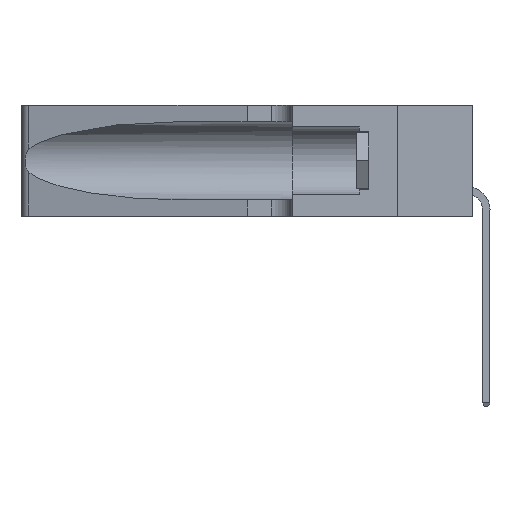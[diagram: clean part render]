
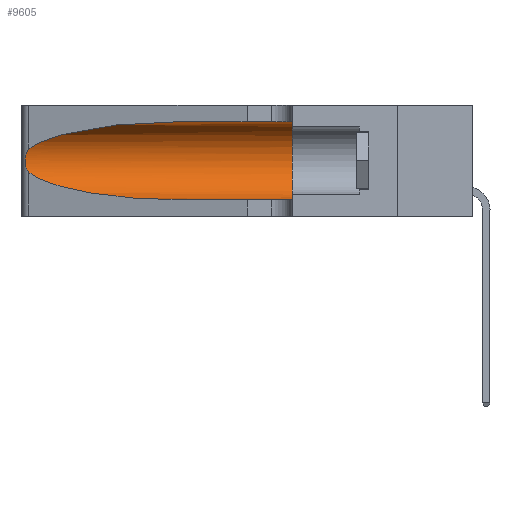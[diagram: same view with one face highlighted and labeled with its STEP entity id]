
A CAD part, left-side view. The second image highlights one B-rep face of the part: STEP entity #9605.
In plain terms, the highlighted cylindrical face has radius 3.308 mm (diameter 6.617 mm), a partial arc.
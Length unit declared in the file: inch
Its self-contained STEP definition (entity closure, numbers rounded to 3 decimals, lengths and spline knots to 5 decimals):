
#351 = CARTESIAN_POINT ( 'NONE',  ( 0.1305, 1.61858, 0.31525 ) ) ;
#369 = CARTESIAN_POINT ( 'NONE',  ( 0.18966, 0.96281, 0.05475 ) ) ;
#580 = VECTOR ( 'NONE', #4025, 39.37008 ) ;
#853 = CARTESIAN_POINT ( 'NONE',  ( 0.1305, 1.61858, 0.05475 ) ) ;
#1292 = CARTESIAN_POINT ( 'NONE',  ( 0.25555, 1.22994, 0.2215 ) ) ;
#1691 = CARTESIAN_POINT ( 'NONE',  ( 0.25487, 1.22718, 0.22369 ) ) ;
#1742 = B_SPLINE_CURVE_WITH_KNOTS ( 'NONE', 3,
 ( #2287, #1292, #12880, #4626, #5923, #19458, #17597, #19232, #20907, #10933, #14302, #15964, #11426, #6297 ),
 .UNSPECIFIED., .F., .F.,
 ( 4, 2, 2, 2, 2, 2, 4 ),
 ( 0., 0.00027, 0.00053, 0.00107, 0.0016, 0.00187, 0.00214 ),
 .UNSPECIFIED. ) ;
#1849 = DIRECTION ( 'NONE',  ( 0., 0., -1. ) ) ;
#1911 = DIRECTION ( 'NONE',  ( 0., -1., 0. ) ) ;
#1985 = CARTESIAN_POINT ( 'NONE',  ( 0.1305, 0.35, 0.05475 ) ) ;
#2013 = ORIENTED_EDGE ( 'NONE', *, *, #16988, .T. ) ;
#2097 = EDGE_CURVE ( 'NONE', #17819, #12978, #13311, .T. ) ;
#2272 = VERTEX_POINT ( 'NONE', #18849 ) ;
#2287 = CARTESIAN_POINT ( 'NONE',  ( 0.25487, 1.22718, 0.22369 ) ) ;
#2636 = ORIENTED_EDGE ( 'NONE', *, *, #2097, .F. ) ;
#3358 = CARTESIAN_POINT ( 'NONE',  ( 0.1305, 0.72297, 0.05475 ) ) ;
#3577 = EDGE_CURVE ( 'NONE', #6447, #12978, #5192, .T. ) ;
#4025 = DIRECTION ( 'NONE',  ( 0., -1., 0. ) ) ;
#4560 = CARTESIAN_POINT ( 'NONE',  ( 0.1305, 0.72297, 0.05475 ) ) ;
#4626 = CARTESIAN_POINT ( 'NONE',  ( 0.25787, 1.23484, 0.2124 ) ) ;
#5049 = CARTESIAN_POINT ( 'NONE',  ( 0.18966, 0.96281, 0.31525 ) ) ;
#5192 = LINE ( 'NONE', #853, #580 ) ;
#5923 = CARTESIAN_POINT ( 'NONE',  ( 0.25854, 1.2359, 0.20912 ) ) ;
#6257 = CARTESIAN_POINT ( 'NONE',  ( 0.1305, 0.35, 0.185 ) ) ;
#6297 = CARTESIAN_POINT ( 'NONE',  ( 0.25487, 1.22718, 0.14631 ) ) ;
#6447 = VERTEX_POINT ( 'NONE', #4560 ) ;
#6607 = DIRECTION ( 'NONE',  ( 0., 0., 1. ) ) ;
#6921 = CARTESIAN_POINT ( 'NONE',  ( 0.2373, 1.15595, 0.08982 ) ) ;
#8172 = CARTESIAN_POINT ( 'NONE',  ( 0.2373, 1.15595, 0.28018 ) ) ;
#9605 = ADVANCED_FACE ( 'NONE', ( #10997 ), #21423, .F. ) ;
#10014 = CARTESIAN_POINT ( 'NONE',  ( 0.1305, 0.72297, 0.31525 ) ) ;
#10046 = ORIENTED_EDGE ( 'NONE', *, *, #14649, .T. ) ;
#10933 = CARTESIAN_POINT ( 'NONE',  ( 0.25856, 1.23593, 0.16098 ) ) ;
#10995 = CARTESIAN_POINT ( 'NONE',  ( 0.1305, 0.35, 0.31525 ) ) ;
#10997 = FACE_OUTER_BOUND ( 'NONE', #14309, .T. ) ;
#11084 = AXIS2_PLACEMENT_3D ( 'NONE', #6257, #17912, #6607 ) ;
#11378 = LINE ( 'NONE', #351, #18455 ) ;
#11426 = CARTESIAN_POINT ( 'NONE',  ( 0.25555, 1.22993, 0.14849 ) ) ;
#11685 = CARTESIAN_POINT ( 'NONE',  ( 0.1305, 1.61858, 0.185 ) ) ;
#11759 = DIRECTION ( 'NONE',  ( 0., -1., 0. ) ) ;
#12246 =( BOUNDED_CURVE ( )  B_SPLINE_CURVE ( 3, ( #18244, #5049, #8172, #16710 ),
 .UNSPECIFIED., .F., .T. ) 
 B_SPLINE_CURVE_WITH_KNOTS ( ( 4, 4 ),
 ( 1.5708, 2.84003 ),
 .UNSPECIFIED. ) 
 CURVE ( )  GEOMETRIC_REPRESENTATION_ITEM ( )  RATIONAL_B_SPLINE_CURVE ( ( 1., 0.87, 0.87, 1. ) ) 
 REPRESENTATION_ITEM ( '' )  );
#12262 = EDGE_CURVE ( 'NONE', #19877, #2272, #1742, .T. ) ;
#12487 = AXIS2_PLACEMENT_3D ( 'NONE', #11685, #11759, #1849 ) ;
#12880 = CARTESIAN_POINT ( 'NONE',  ( 0.25639, 1.23184, 0.21858 ) ) ;
#12966 = EDGE_CURVE ( 'NONE', #16226, #17819, #11378, .T. ) ;
#12978 = VERTEX_POINT ( 'NONE', #1985 ) ;
#13306 = CARTESIAN_POINT ( 'NONE',  ( 0.25487, 1.22718, 0.14631 ) ) ;
#13311 = CIRCLE ( 'NONE', #11084, 0.13025 ) ;
#14302 = CARTESIAN_POINT ( 'NONE',  ( 0.25789, 1.23486, 0.15765 ) ) ;
#14309 = EDGE_LOOP ( 'NONE', ( #10046, #19003, #2013, #17803, #2636, #19685 ) ) ;
#14649 = EDGE_CURVE ( 'NONE', #16226, #19877, #12246, .T. ) ;
#15964 = CARTESIAN_POINT ( 'NONE',  ( 0.25639, 1.23186, 0.15144 ) ) ;
#16226 = VERTEX_POINT ( 'NONE', #10014 ) ;
#16710 = CARTESIAN_POINT ( 'NONE',  ( 0.25487, 1.22718, 0.22369 ) ) ;
#16988 = EDGE_CURVE ( 'NONE', #2272, #6447, #20000, .T. ) ;
#17597 = CARTESIAN_POINT ( 'NONE',  ( 0.26075, 1.23896, 0.19203 ) ) ;
#17803 = ORIENTED_EDGE ( 'NONE', *, *, #3577, .T. ) ;
#17819 = VERTEX_POINT ( 'NONE', #10995 ) ;
#17912 = DIRECTION ( 'NONE',  ( 0., 1., 0. ) ) ;
#18244 = CARTESIAN_POINT ( 'NONE',  ( 0.1305, 0.72297, 0.31525 ) ) ;
#18455 = VECTOR ( 'NONE', #1911, 39.37008 ) ;
#18849 = CARTESIAN_POINT ( 'NONE',  ( 0.25487, 1.22718, 0.14631 ) ) ;
#19003 = ORIENTED_EDGE ( 'NONE', *, *, #12262, .T. ) ;
#19232 = CARTESIAN_POINT ( 'NONE',  ( 0.26075, 1.23896, 0.178 ) ) ;
#19458 = CARTESIAN_POINT ( 'NONE',  ( 0.26018, 1.23835, 0.19895 ) ) ;
#19685 = ORIENTED_EDGE ( 'NONE', *, *, #12966, .F. ) ;
#19877 = VERTEX_POINT ( 'NONE', #1691 ) ;
#20000 =( BOUNDED_CURVE ( )  B_SPLINE_CURVE ( 3, ( #13306, #6921, #369, #3358 ),
 .UNSPECIFIED., .F., .F. ) 
 B_SPLINE_CURVE_WITH_KNOTS ( ( 4, 4 ),
 ( 3.44316, 4.71239 ),
 .UNSPECIFIED. ) 
 CURVE ( )  GEOMETRIC_REPRESENTATION_ITEM ( )  RATIONAL_B_SPLINE_CURVE ( ( 1., 0.87, 0.87, 1. ) ) 
 REPRESENTATION_ITEM ( '' )  );
#20907 = CARTESIAN_POINT ( 'NONE',  ( 0.26017, 1.23833, 0.17102 ) ) ;
#21423 = CYLINDRICAL_SURFACE ( 'NONE', #12487, 0.13025 ) ;
